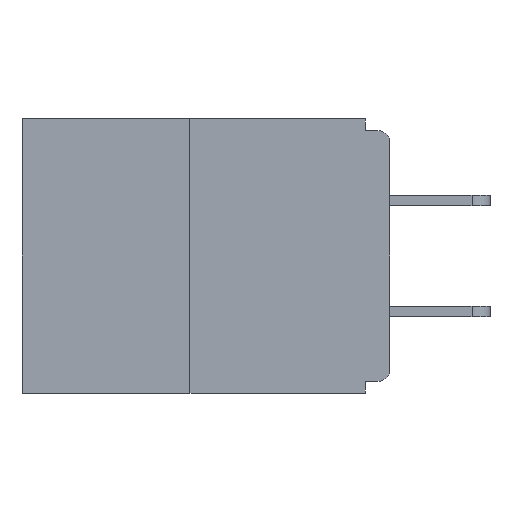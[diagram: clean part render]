
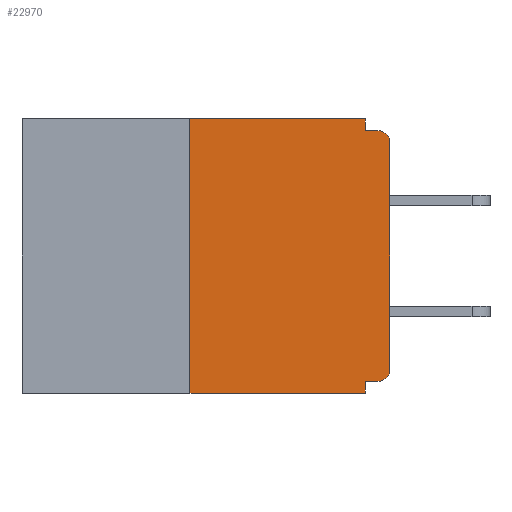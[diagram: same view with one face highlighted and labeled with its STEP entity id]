
A CAD part, left-side view. The second image highlights one B-rep face of the part: STEP entity #22970.
In plain terms, the highlighted planar face has unit normal (-1, 0, 0).
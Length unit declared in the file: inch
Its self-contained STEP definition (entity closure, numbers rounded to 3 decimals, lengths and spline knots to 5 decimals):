
#306 = CARTESIAN_POINT ( 'NONE',  ( 0., 0., -0.313 ) ) ;
#670 = VERTEX_POINT ( 'NONE', #16619 ) ;
#946 = VECTOR ( 'NONE', #26239, 39.37008 ) ;
#1028 = LINE ( 'NONE', #3929, #6023 ) ;
#1286 = EDGE_CURVE ( 'NONE', #11219, #22699, #11641, .T. ) ;
#1525 = VERTEX_POINT ( 'NONE', #306 ) ;
#1738 = VERTEX_POINT ( 'NONE', #20623 ) ;
#2317 = EDGE_CURVE ( 'NONE', #20714, #670, #4502, .T. ) ;
#2399 = AXIS2_PLACEMENT_3D ( 'NONE', #24914, #9227, #27302 ) ;
#3486 = CARTESIAN_POINT ( 'NONE',  ( 0., 0.25, -0.343 ) ) ;
#3929 = CARTESIAN_POINT ( 'NONE',  ( 0., 0.46, 0. ) ) ;
#4502 = LINE ( 'NONE', #12790, #5195 ) ;
#4801 = LINE ( 'NONE', #21156, #27164 ) ;
#4861 = DIRECTION ( 'NONE',  ( -1., 0., 0. ) ) ;
#5195 = VECTOR ( 'NONE', #28705, 39.37008 ) ;
#5612 = VERTEX_POINT ( 'NONE', #26251 ) ;
#6009 = ORIENTED_EDGE ( 'NONE', *, *, #9085, .F. ) ;
#6023 = VECTOR ( 'NONE', #8149, 39.37008 ) ;
#6224 = CIRCLE ( 'NONE', #2399, 0.015 ) ;
#6665 = CARTESIAN_POINT ( 'NONE',  ( 0., 0., 0. ) ) ;
#7267 = EDGE_CURVE ( 'NONE', #1738, #20714, #24876, .T. ) ;
#7858 = ORIENTED_EDGE ( 'NONE', *, *, #8089, .F. ) ;
#8007 = DIRECTION ( 'NONE',  ( 0., 0., -1. ) ) ;
#8089 = EDGE_CURVE ( 'NONE', #25862, #1738, #1028, .T. ) ;
#8149 = DIRECTION ( 'NONE',  ( 0., -1., 0. ) ) ;
#8366 = PLANE ( 'NONE',  #25639 ) ;
#8523 = ORIENTED_EDGE ( 'NONE', *, *, #7267, .F. ) ;
#9085 = EDGE_CURVE ( 'NONE', #24975, #22699, #14092, .T. ) ;
#9227 = DIRECTION ( 'NONE',  ( -1., 0., 0. ) ) ;
#9278 = ORIENTED_EDGE ( 'NONE', *, *, #21237, .F. ) ;
#9456 = DIRECTION ( 'NONE',  ( 0., 1., 0. ) ) ;
#9980 = LINE ( 'NONE', #18403, #29195 ) ;
#10794 = CARTESIAN_POINT ( 'NONE',  ( 0., 0.015, -0.328 ) ) ;
#10821 = ORIENTED_EDGE ( 'NONE', *, *, #16123, .F. ) ;
#10975 = ORIENTED_EDGE ( 'NONE', *, *, #26504, .T. ) ;
#11004 = VECTOR ( 'NONE', #8007, 39.37008 ) ;
#11219 = VERTEX_POINT ( 'NONE', #3486 ) ;
#11641 = LINE ( 'NONE', #19246, #27269 ) ;
#11857 = CARTESIAN_POINT ( 'NONE',  ( 0., 0.031, -0.015 ) ) ;
#12790 = CARTESIAN_POINT ( 'NONE',  ( 0., 0., -0.015 ) ) ;
#14092 = LINE ( 'NONE', #14935, #946 ) ;
#14175 = EDGE_CURVE ( 'NONE', #1525, #5612, #16983, .T. ) ;
#14935 = CARTESIAN_POINT ( 'NONE',  ( 0., 0.031, -0.343 ) ) ;
#15211 = ORIENTED_EDGE ( 'NONE', *, *, #2317, .F. ) ;
#15233 = DIRECTION ( 'NONE',  ( 1., 0., 0. ) ) ;
#15322 = DIRECTION ( 'NONE',  ( 0., 0., -1. ) ) ;
#16123 = EDGE_CURVE ( 'NONE', #11219, #25862, #4801, .T. ) ;
#16523 = EDGE_LOOP ( 'NONE', ( #7858, #10821, #23740, #6009, #9278, #17082, #21157, #10975, #15211, #8523 ) ) ;
#16619 = CARTESIAN_POINT ( 'NONE',  ( 0., 0.015, -0.015 ) ) ;
#16983 = LINE ( 'NONE', #6665, #18025 ) ;
#17022 = CARTESIAN_POINT ( 'NONE',  ( 0., 0.031, -0.328 ) ) ;
#17062 = DIRECTION ( 'NONE',  ( 0., -1., 0. ) ) ;
#17082 = ORIENTED_EDGE ( 'NONE', *, *, #17521, .T. ) ;
#17521 = EDGE_CURVE ( 'NONE', #18276, #1525, #23901, .T. ) ;
#17701 = CARTESIAN_POINT ( 'NONE',  ( 0., 0.25, 0. ) ) ;
#18025 = VECTOR ( 'NONE', #22321, 39.37008 ) ;
#18276 = VERTEX_POINT ( 'NONE', #10794 ) ;
#18403 = CARTESIAN_POINT ( 'NONE',  ( 0., 0., -0.328 ) ) ;
#18452 = CARTESIAN_POINT ( 'NONE',  ( 0., 0.015, -0.313 ) ) ;
#19246 = CARTESIAN_POINT ( 'NONE',  ( 0., 0.46, -0.343 ) ) ;
#20623 = CARTESIAN_POINT ( 'NONE',  ( 0., 0.031, 0. ) ) ;
#20714 = VERTEX_POINT ( 'NONE', #11857 ) ;
#21156 = CARTESIAN_POINT ( 'NONE',  ( 0., 0.25, 0. ) ) ;
#21157 = ORIENTED_EDGE ( 'NONE', *, *, #14175, .T. ) ;
#21237 = EDGE_CURVE ( 'NONE', #18276, #24975, #9980, .T. ) ;
#21602 = CARTESIAN_POINT ( 'NONE',  ( 0., 0.031, 0. ) ) ;
#21807 = CARTESIAN_POINT ( 'NONE',  ( 0., 0.031, -0.343 ) ) ;
#21999 = AXIS2_PLACEMENT_3D ( 'NONE', #18452, #4861, #23016 ) ;
#22321 = DIRECTION ( 'NONE',  ( 0., 0., 1. ) ) ;
#22699 = VERTEX_POINT ( 'NONE', #21807 ) ;
#22970 = ADVANCED_FACE ( 'NONE', ( #23050 ), #8366, .F. ) ;
#23016 = DIRECTION ( 'NONE',  ( 0., 0., -1. ) ) ;
#23050 = FACE_OUTER_BOUND ( 'NONE', #16523, .T. ) ;
#23523 = DIRECTION ( 'NONE',  ( 0., 0., 1. ) ) ;
#23740 = ORIENTED_EDGE ( 'NONE', *, *, #1286, .T. ) ;
#23901 = CIRCLE ( 'NONE', #21999, 0.015 ) ;
#24876 = LINE ( 'NONE', #21602, #11004 ) ;
#24914 = CARTESIAN_POINT ( 'NONE',  ( 0., 0.015, -0.03 ) ) ;
#24975 = VERTEX_POINT ( 'NONE', #17022 ) ;
#25639 = AXIS2_PLACEMENT_3D ( 'NONE', #28845, #15233, #15322 ) ;
#25862 = VERTEX_POINT ( 'NONE', #17701 ) ;
#26239 = DIRECTION ( 'NONE',  ( 0., 0., -1. ) ) ;
#26251 = CARTESIAN_POINT ( 'NONE',  ( 0., 0., -0.03 ) ) ;
#26504 = EDGE_CURVE ( 'NONE', #5612, #670, #6224, .T. ) ;
#27164 = VECTOR ( 'NONE', #23523, 39.37008 ) ;
#27269 = VECTOR ( 'NONE', #17062, 39.37008 ) ;
#27302 = DIRECTION ( 'NONE',  ( 0., 0., -1. ) ) ;
#28705 = DIRECTION ( 'NONE',  ( 0., -1., 0. ) ) ;
#28845 = CARTESIAN_POINT ( 'NONE',  ( 0., 0.46, 0. ) ) ;
#29195 = VECTOR ( 'NONE', #9456, 39.37008 ) ;
